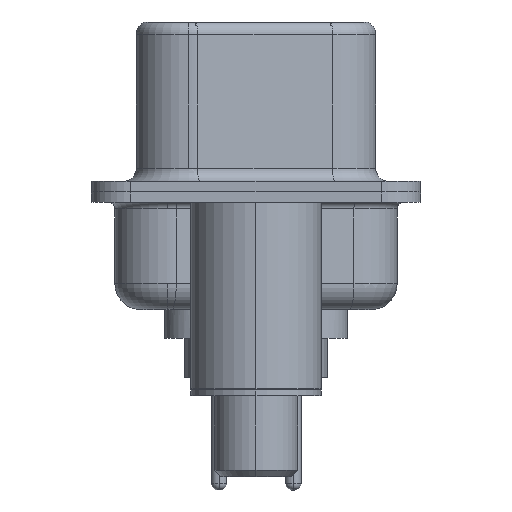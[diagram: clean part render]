
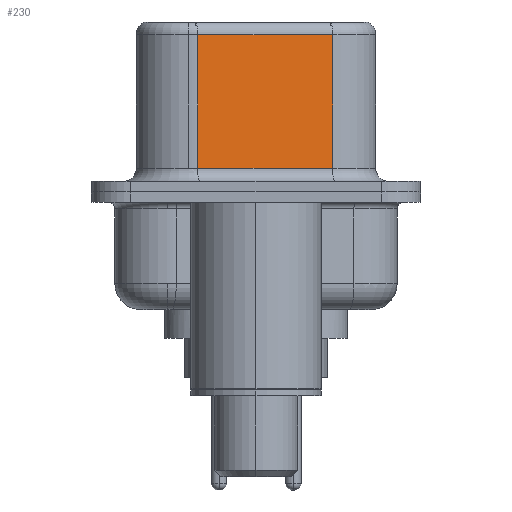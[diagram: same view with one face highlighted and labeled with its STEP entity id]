
A CAD part, left-side view. The second image highlights one B-rep face of the part: STEP entity #230.
In plain terms, the highlighted planar face has unit normal (-0.985, -0.174, 0).
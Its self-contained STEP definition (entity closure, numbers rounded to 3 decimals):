
#230 = ADVANCED_FACE ( 'NONE', ( #17291 ), #7771, .F. ) ;
#331 = CARTESIAN_POINT ( 'NONE',  ( 3.67, 2.233, 0.9 ) ) ;
#380 = ORIENTED_EDGE ( 'NONE', *, *, #10976, .T. ) ;
#1149 = ORIENTED_EDGE ( 'NONE', *, *, #7240, .T. ) ;
#1320 = VECTOR ( 'NONE', #13904, 1000. ) ;
#2575 = DIRECTION ( 'NONE',  ( 0.174, -0.985, 0. ) ) ;
#2676 = CARTESIAN_POINT ( 'NONE',  ( 4.58, -2.927, 0.9 ) ) ;
#2926 = VERTEX_POINT ( 'NONE', #14441 ) ;
#3048 = ORIENTED_EDGE ( 'NONE', *, *, #7632, .F. ) ;
#3768 = DIRECTION ( 'NONE',  ( 0.985, 0.174, 0. ) ) ;
#3877 = LINE ( 'NONE', #9399, #7490 ) ;
#4006 = LINE ( 'NONE', #11338, #15558 ) ;
#5872 = ORIENTED_EDGE ( 'NONE', *, *, #8701, .T. ) ;
#6572 = LINE ( 'NONE', #13184, #18119 ) ;
#7240 = EDGE_CURVE ( 'NONE', #14469, #9043, #6572, .T. ) ;
#7490 = VECTOR ( 'NONE', #13881, 1000. ) ;
#7632 = EDGE_CURVE ( 'NONE', #2926, #9043, #3877, .T. ) ;
#7771 = PLANE ( 'NONE',  #10268 ) ;
#7938 = CARTESIAN_POINT ( 'NONE',  ( 4.58, -2.927, 6.52 ) ) ;
#8701 = EDGE_CURVE ( 'NONE', #19436, #14469, #17604, .T. ) ;
#9043 = VERTEX_POINT ( 'NONE', #2676 ) ;
#9399 = CARTESIAN_POINT ( 'NONE',  ( 4.58, -2.927, 6.52 ) ) ;
#9829 = DIRECTION ( 'NONE',  ( -0.174, 0.985, 0. ) ) ;
#9971 = DIRECTION ( 'NONE',  ( -0.174, 0.985, 0. ) ) ;
#10268 = AXIS2_PLACEMENT_3D ( 'NONE', #7938, #3768, #9971 ) ;
#10976 = EDGE_CURVE ( 'NONE', #2926, #19436, #4006, .T. ) ;
#11338 = CARTESIAN_POINT ( 'NONE',  ( 4.58, -2.927, 6.02 ) ) ;
#12365 = CARTESIAN_POINT ( 'NONE',  ( 3.67, 2.233, 6.52 ) ) ;
#13184 = CARTESIAN_POINT ( 'NONE',  ( 4.58, -2.927, 0.9 ) ) ;
#13881 = DIRECTION ( 'NONE',  ( 0., 0., -1. ) ) ;
#13904 = DIRECTION ( 'NONE',  ( 0., 0., -1. ) ) ;
#14441 = CARTESIAN_POINT ( 'NONE',  ( 4.58, -2.927, 6.02 ) ) ;
#14469 = VERTEX_POINT ( 'NONE', #331 ) ;
#15558 = VECTOR ( 'NONE', #9829, 1000. ) ;
#15616 = CARTESIAN_POINT ( 'NONE',  ( 3.67, 2.233, 6.02 ) ) ;
#17291 = FACE_OUTER_BOUND ( 'NONE', #17903, .T. ) ;
#17604 = LINE ( 'NONE', #12365, #1320 ) ;
#17903 = EDGE_LOOP ( 'NONE', ( #3048, #380, #5872, #1149 ) ) ;
#18119 = VECTOR ( 'NONE', #2575, 1000. ) ;
#19436 = VERTEX_POINT ( 'NONE', #15616 ) ;
